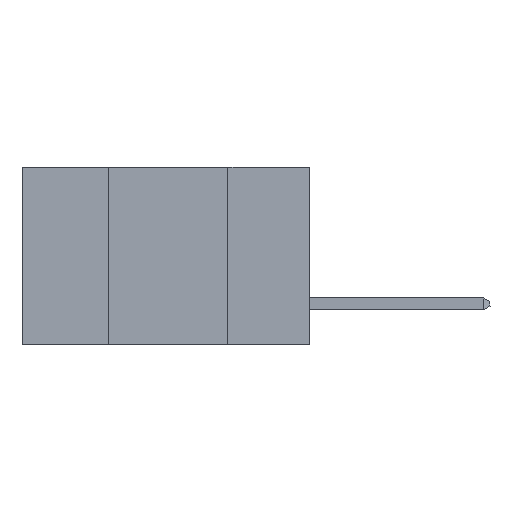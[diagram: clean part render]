
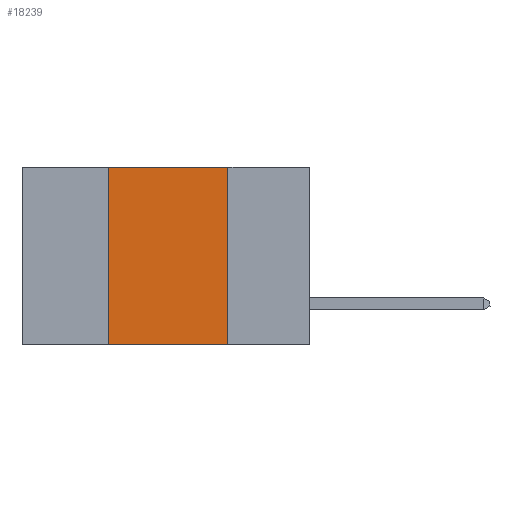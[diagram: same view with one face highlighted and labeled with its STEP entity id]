
A CAD part, left-side view. The second image highlights one B-rep face of the part: STEP entity #18239.
In plain terms, the highlighted planar face has unit normal (-1, 0, 0).
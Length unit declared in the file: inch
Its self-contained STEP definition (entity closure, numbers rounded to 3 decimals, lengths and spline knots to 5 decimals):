
#103 = CARTESIAN_POINT ( 'NONE',  ( 0., 0.6, 0. ) ) ;
#182 = VECTOR ( 'NONE', #13987, 39.37008 ) ;
#261 = ORIENTED_EDGE ( 'NONE', *, *, #15804, .F. ) ;
#491 = EDGE_CURVE ( 'NONE', #9140, #18524, #19521, .T. ) ;
#1298 = LINE ( 'NONE', #103, #12307 ) ;
#1979 = EDGE_CURVE ( 'NONE', #12746, #18524, #16968, .T. ) ;
#2356 = CARTESIAN_POINT ( 'NONE',  ( 0., 0.17, 0. ) ) ;
#2791 = ORIENTED_EDGE ( 'NONE', *, *, #1979, .T. ) ;
#3619 = ORIENTED_EDGE ( 'NONE', *, *, #491, .F. ) ;
#4736 = VECTOR ( 'NONE', #19091, 39.37008 ) ;
#5016 = DIRECTION ( 'NONE',  ( 1., 0., 0. ) ) ;
#6420 = VERTEX_POINT ( 'NONE', #11078 ) ;
#7637 = CARTESIAN_POINT ( 'NONE',  ( 0., 0.17, -0.37 ) ) ;
#8162 = DIRECTION ( 'NONE',  ( 0., -1., 0. ) ) ;
#8662 = FACE_OUTER_BOUND ( 'NONE', #16697, .T. ) ;
#9140 = VERTEX_POINT ( 'NONE', #2356 ) ;
#9212 = CARTESIAN_POINT ( 'NONE',  ( 0., 0.42, -0.37 ) ) ;
#9787 = DIRECTION ( 'NONE',  ( 0., 0., -1. ) ) ;
#11078 = CARTESIAN_POINT ( 'NONE',  ( 0., 0.42, 0. ) ) ;
#12307 = VECTOR ( 'NONE', #8162, 39.37008 ) ;
#12387 = CARTESIAN_POINT ( 'NONE',  ( 0., 0.17, 0. ) ) ;
#12461 = CARTESIAN_POINT ( 'NONE',  ( 0., 0.42, 0. ) ) ;
#12746 = VERTEX_POINT ( 'NONE', #9212 ) ;
#13987 = DIRECTION ( 'NONE',  ( 0., 0., 1. ) ) ;
#14224 = PLANE ( 'NONE',  #16734 ) ;
#14793 = CARTESIAN_POINT ( 'NONE',  ( 0., 0.6, -0.37 ) ) ;
#15766 = DIRECTION ( 'NONE',  ( 0., 0., -1. ) ) ;
#15804 = EDGE_CURVE ( 'NONE', #6420, #9140, #1298, .T. ) ;
#16290 = LINE ( 'NONE', #12461, #182 ) ;
#16352 = ORIENTED_EDGE ( 'NONE', *, *, #17517, .F. ) ;
#16697 = EDGE_LOOP ( 'NONE', ( #3619, #261, #16352, #2791 ) ) ;
#16734 = AXIS2_PLACEMENT_3D ( 'NONE', #17209, #5016, #15766 ) ;
#16968 = LINE ( 'NONE', #14793, #4736 ) ;
#17209 = CARTESIAN_POINT ( 'NONE',  ( 0., 0.6, 0. ) ) ;
#17517 = EDGE_CURVE ( 'NONE', #12746, #6420, #16290, .T. ) ;
#18239 = ADVANCED_FACE ( 'NONE', ( #8662 ), #14224, .F. ) ;
#18524 = VERTEX_POINT ( 'NONE', #7637 ) ;
#19090 = VECTOR ( 'NONE', #9787, 39.37008 ) ;
#19091 = DIRECTION ( 'NONE',  ( 0., -1., 0. ) ) ;
#19521 = LINE ( 'NONE', #12387, #19090 ) ;
